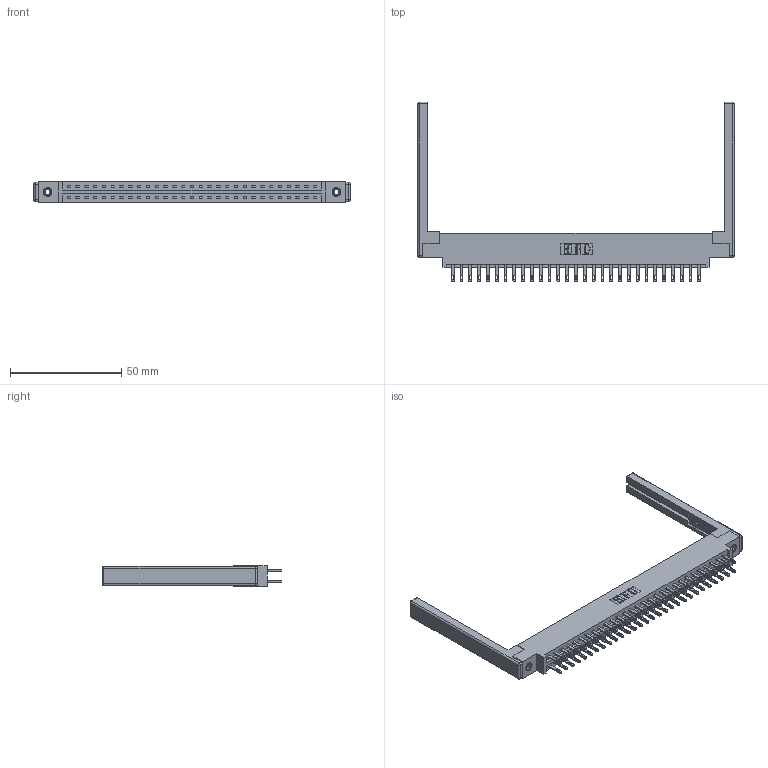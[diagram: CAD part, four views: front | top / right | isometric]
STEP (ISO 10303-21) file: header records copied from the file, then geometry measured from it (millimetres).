
FILE_DESCRIPTION (( 'STEP AP203' ), '1' );
FILE_NAME ('337-058-500-868.STEP', '2019-10-11T20:23:38', ( '' ), ( '' ), 'SwSTEP 2.0', 'SolidWorks 2016', '' );
FILE_SCHEMA (( 'CONFIG_CONTROL_DESIGN' ));
Length unit declared in the file: inch
Products named in the file (5): 345-292-001_345-293-100; 337-058-500-868; 307-220-068; 337 Part_0.170 Offset - 0.156 Dia-TI; 345-250-001_345-250-001-102
Assembly tree (63 placements, depth 2):
  337-058-500-868
    337 Part_0.170 Offset - 0.156 Dia-TI
    345-292-001_345-293-100  x58
    345-250-001_345-250-001-102  x2
    307-220-068  x2
Bounding box: 142.34 x 80.9 x 9.4 mm (x, y, z)
Volume: 19272.6 mm3; surface area: 21490.1 mm2
Topology: 63 solids, 63 shells, 3172 faces, 9587 edges, 6370 vertices
Faces by surface type: plane 2018, cylinder 1130, cone 12, sphere 8, torus 4
Entity records: 26988 total; most frequent: CARTESIAN_POINT 4523, ORIENTED_EDGE 4448, DIRECTION 3942, EDGE_CURVE 2224, VECTOR 2042, LINE 2042, VERTEX_POINT 1474, AXIS2_PLACEMENT_3D 950
